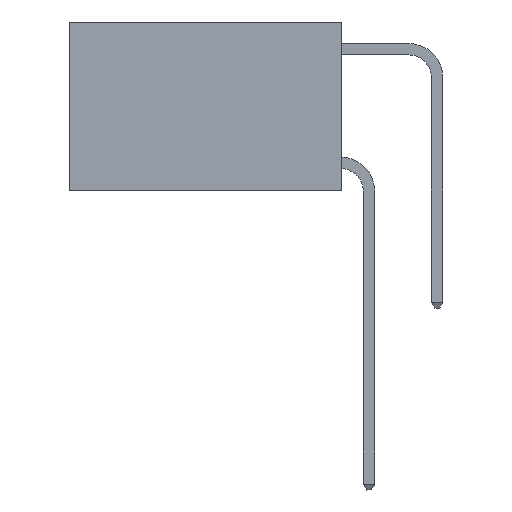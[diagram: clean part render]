
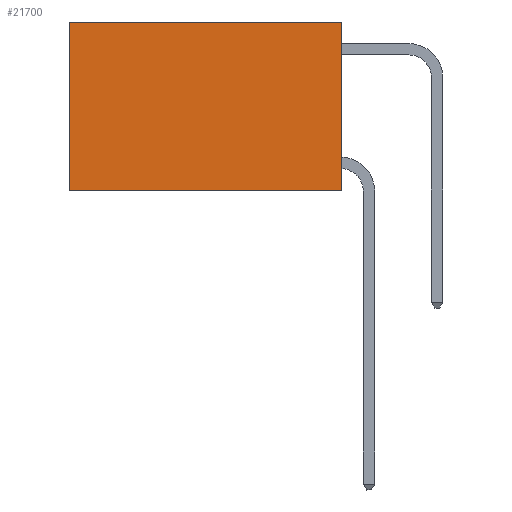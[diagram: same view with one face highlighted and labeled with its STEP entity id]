
A CAD part, left-side view. The second image highlights one B-rep face of the part: STEP entity #21700.
In plain terms, the highlighted planar face has unit normal (-1, 0, 0).
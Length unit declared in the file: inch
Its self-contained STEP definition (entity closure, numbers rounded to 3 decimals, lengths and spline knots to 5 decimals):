
#591 = ORIENTED_EDGE ( 'NONE', *, *, #18589, .F. ) ;
#1186 = LINE ( 'NONE', #14997, #16313 ) ;
#4307 = PLANE ( 'NONE',  #25293 ) ;
#4382 = EDGE_LOOP ( 'NONE', ( #5165, #21887, #591, #13045 ) ) ;
#4586 = VERTEX_POINT ( 'NONE', #17589 ) ;
#5165 = ORIENTED_EDGE ( 'NONE', *, *, #16191, .T. ) ;
#5247 = CARTESIAN_POINT ( 'NONE',  ( 0.2625, 0., 0. ) ) ;
#7674 = EDGE_CURVE ( 'NONE', #12940, #4586, #25335, .T. ) ;
#9233 = CARTESIAN_POINT ( 'NONE',  ( 0.2625, 0., 0. ) ) ;
#10100 = CARTESIAN_POINT ( 'NONE',  ( 0.2625, 0., 0. ) ) ;
#11092 = DIRECTION ( 'NONE',  ( 1., 0., 0. ) ) ;
#12319 = VECTOR ( 'NONE', #14390, 39.37008 ) ;
#12940 = VERTEX_POINT ( 'NONE', #9233 ) ;
#13032 = LINE ( 'NONE', #5247, #12319 ) ;
#13045 = ORIENTED_EDGE ( 'NONE', *, *, #7674, .T. ) ;
#13480 = VECTOR ( 'NONE', #14593, 39.37008 ) ;
#14390 = DIRECTION ( 'NONE',  ( 0., 0., -1. ) ) ;
#14593 = DIRECTION ( 'NONE',  ( 0., 1., 0. ) ) ;
#14997 = CARTESIAN_POINT ( 'NONE',  ( 0.2625, 0., -0.37 ) ) ;
#15450 = CARTESIAN_POINT ( 'NONE',  ( 0.2625, 0.6, -0.37 ) ) ;
#16191 = EDGE_CURVE ( 'NONE', #4586, #22943, #25763, .T. ) ;
#16313 = VECTOR ( 'NONE', #28275, 39.37008 ) ;
#16760 = CARTESIAN_POINT ( 'NONE',  ( 0.2625, 0., -0.37 ) ) ;
#16958 = CARTESIAN_POINT ( 'NONE',  ( 0.2625, 0.6, 0. ) ) ;
#17589 = CARTESIAN_POINT ( 'NONE',  ( 0.2625, 0.6, 0. ) ) ;
#18589 = EDGE_CURVE ( 'NONE', #12940, #26612, #13032, .T. ) ;
#19858 = VECTOR ( 'NONE', #21454, 39.37008 ) ;
#21454 = DIRECTION ( 'NONE',  ( 0., 0., -1. ) ) ;
#21700 = ADVANCED_FACE ( 'NONE', ( #25122 ), #4307, .F. ) ;
#21887 = ORIENTED_EDGE ( 'NONE', *, *, #25503, .F. ) ;
#22943 = VERTEX_POINT ( 'NONE', #15450 ) ;
#24377 = CARTESIAN_POINT ( 'NONE',  ( 0.2625, 0., 0. ) ) ;
#25122 = FACE_OUTER_BOUND ( 'NONE', #4382, .T. ) ;
#25293 = AXIS2_PLACEMENT_3D ( 'NONE', #24377, #11092, #26684 ) ;
#25335 = LINE ( 'NONE', #10100, #13480 ) ;
#25503 = EDGE_CURVE ( 'NONE', #26612, #22943, #1186, .T. ) ;
#25763 = LINE ( 'NONE', #16958, #19858 ) ;
#26612 = VERTEX_POINT ( 'NONE', #16760 ) ;
#26684 = DIRECTION ( 'NONE',  ( 0., 0., -1. ) ) ;
#28275 = DIRECTION ( 'NONE',  ( 0., 1., 0. ) ) ;
